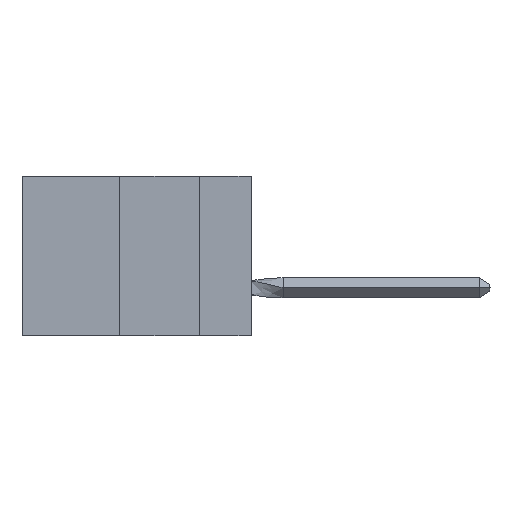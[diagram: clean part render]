
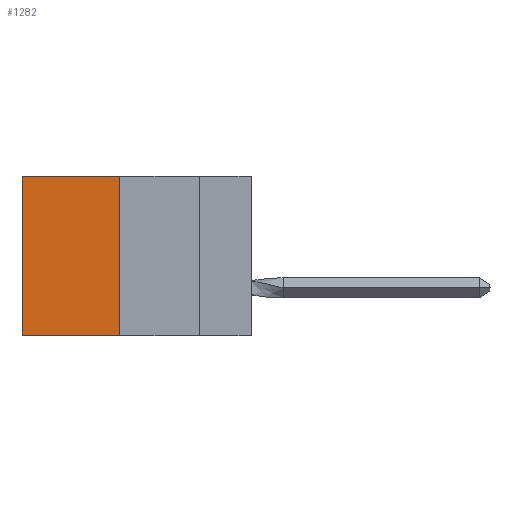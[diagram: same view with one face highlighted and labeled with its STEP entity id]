
A CAD part, left-side view. The second image highlights one B-rep face of the part: STEP entity #1282.
In plain terms, the highlighted planar face has unit normal (-1, 0, 0).
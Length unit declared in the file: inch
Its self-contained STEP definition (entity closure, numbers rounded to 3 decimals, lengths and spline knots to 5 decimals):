
#239 = CARTESIAN_POINT ( 'NONE',  ( 0.305, 0.413, 0. ) ) ;
#1078 = FACE_OUTER_BOUND ( 'NONE', #20730, .T. ) ;
#1282 = ADVANCED_FACE ( 'NONE', ( #1078 ), #14489, .F. ) ;
#2295 = VECTOR ( 'NONE', #12775, 39.37008 ) ;
#2465 = LINE ( 'NONE', #17319, #12298 ) ;
#2538 = LINE ( 'NONE', #239, #8230 ) ;
#3073 = DIRECTION ( 'NONE',  ( 0., 0., -1. ) ) ;
#4088 = CARTESIAN_POINT ( 'NONE',  ( 0.305, 0.413, 0. ) ) ;
#4729 = CARTESIAN_POINT ( 'NONE',  ( 0.305, 0.413, -0.5 ) ) ;
#5668 = DIRECTION ( 'NONE',  ( 0., 1., 0. ) ) ;
#6314 = VERTEX_POINT ( 'NONE', #21058 ) ;
#6326 = VECTOR ( 'NONE', #3073, 39.37008 ) ;
#7217 = LINE ( 'NONE', #13963, #2295 ) ;
#7630 = AXIS2_PLACEMENT_3D ( 'NONE', #4729, #16169, #16028 ) ;
#8230 = VECTOR ( 'NONE', #10955, 39.37008 ) ;
#8788 = ORIENTED_EDGE ( 'NONE', *, *, #10093, .T. ) ;
#9811 = EDGE_CURVE ( 'NONE', #6314, #16456, #7217, .T. ) ;
#10093 = EDGE_CURVE ( 'NONE', #21227, #6314, #2538, .T. ) ;
#10210 = LINE ( 'NONE', #11256, #6326 ) ;
#10420 = CARTESIAN_POINT ( 'NONE',  ( 0.305, 0.72, -0.5 ) ) ;
#10955 = DIRECTION ( 'NONE',  ( 0., 1., 0. ) ) ;
#11256 = CARTESIAN_POINT ( 'NONE',  ( 0.305, 0.413, -0.5 ) ) ;
#11530 = ORIENTED_EDGE ( 'NONE', *, *, #14484, .F. ) ;
#11976 = ORIENTED_EDGE ( 'NONE', *, *, #9811, .T. ) ;
#12298 = VECTOR ( 'NONE', #5668, 39.37008 ) ;
#12775 = DIRECTION ( 'NONE',  ( 0., 0., -1. ) ) ;
#13963 = CARTESIAN_POINT ( 'NONE',  ( 0.305, 0.72, -0.5 ) ) ;
#14484 = EDGE_CURVE ( 'NONE', #21227, #14719, #10210, .T. ) ;
#14489 = PLANE ( 'NONE',  #7630 ) ;
#14719 = VERTEX_POINT ( 'NONE', #18675 ) ;
#15184 = ORIENTED_EDGE ( 'NONE', *, *, #20004, .F. ) ;
#16028 = DIRECTION ( 'NONE',  ( 0., 0., -1. ) ) ;
#16169 = DIRECTION ( 'NONE',  ( 1., 0., 0. ) ) ;
#16456 = VERTEX_POINT ( 'NONE', #10420 ) ;
#17319 = CARTESIAN_POINT ( 'NONE',  ( 0.305, 0.413, -0.5 ) ) ;
#18675 = CARTESIAN_POINT ( 'NONE',  ( 0.305, 0.413, -0.5 ) ) ;
#20004 = EDGE_CURVE ( 'NONE', #14719, #16456, #2465, .T. ) ;
#20730 = EDGE_LOOP ( 'NONE', ( #11976, #15184, #11530, #8788 ) ) ;
#21058 = CARTESIAN_POINT ( 'NONE',  ( 0.305, 0.72, 0. ) ) ;
#21227 = VERTEX_POINT ( 'NONE', #4088 ) ;
